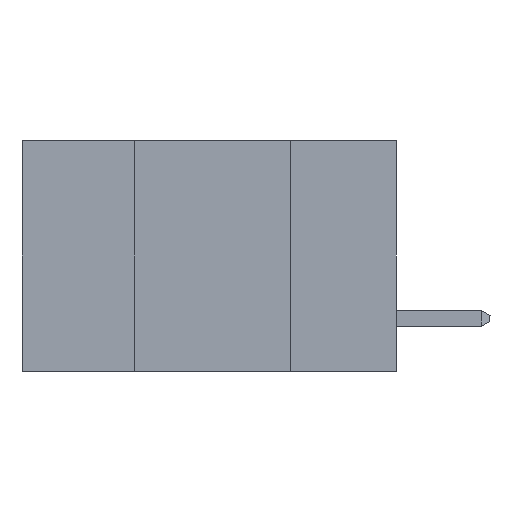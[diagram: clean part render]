
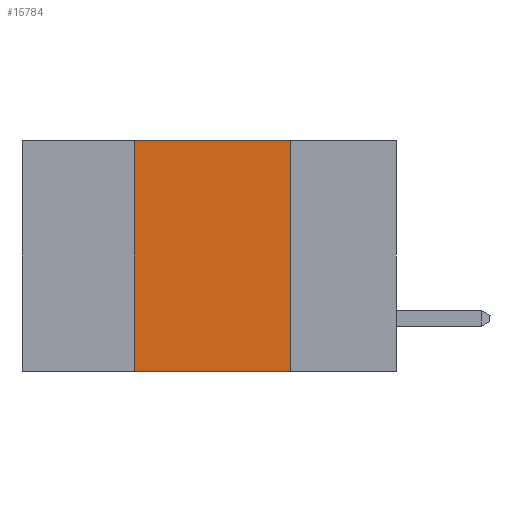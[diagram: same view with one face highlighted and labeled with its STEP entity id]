
A CAD part, left-side view. The second image highlights one B-rep face of the part: STEP entity #15784.
In plain terms, the highlighted planar face has unit normal (-1, 0, 0).
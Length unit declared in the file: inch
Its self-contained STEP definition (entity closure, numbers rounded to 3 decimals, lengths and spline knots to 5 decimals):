
#349 = DIRECTION ( 'NONE',  ( 0., 0., -1. ) ) ;
#464 = CARTESIAN_POINT ( 'NONE',  ( 0., 0.17, 0. ) ) ;
#780 = VERTEX_POINT ( 'NONE', #19838 ) ;
#867 = EDGE_CURVE ( 'NONE', #8004, #780, #4786, .T. ) ;
#2252 = VERTEX_POINT ( 'NONE', #4453 ) ;
#2405 = ORIENTED_EDGE ( 'NONE', *, *, #23906, .F. ) ;
#3900 = VECTOR ( 'NONE', #13728, 39.37008 ) ;
#4453 = CARTESIAN_POINT ( 'NONE',  ( 0., 0.42, 0. ) ) ;
#4786 = LINE ( 'NONE', #6362, #9946 ) ;
#6202 = VECTOR ( 'NONE', #10086, 39.37008 ) ;
#6362 = CARTESIAN_POINT ( 'NONE',  ( 0., 0.6, -0.37 ) ) ;
#6601 = CARTESIAN_POINT ( 'NONE',  ( 0., 0.42, -0.37 ) ) ;
#8004 = VERTEX_POINT ( 'NONE', #6601 ) ;
#8180 = PLANE ( 'NONE',  #9452 ) ;
#8631 = DIRECTION ( 'NONE',  ( 0., -1., 0. ) ) ;
#9372 = ORIENTED_EDGE ( 'NONE', *, *, #14636, .F. ) ;
#9452 = AXIS2_PLACEMENT_3D ( 'NONE', #23384, #12071, #349 ) ;
#9469 = EDGE_CURVE ( 'NONE', #20198, #780, #18580, .T. ) ;
#9946 = VECTOR ( 'NONE', #8631, 39.37008 ) ;
#10086 = DIRECTION ( 'NONE',  ( 0., -1., 0. ) ) ;
#11577 = FACE_OUTER_BOUND ( 'NONE', #12128, .T. ) ;
#12026 = DIRECTION ( 'NONE',  ( 0., 0., -1. ) ) ;
#12071 = DIRECTION ( 'NONE',  ( 1., 0., 0. ) ) ;
#12128 = EDGE_LOOP ( 'NONE', ( #14836, #2405, #9372, #17763 ) ) ;
#12157 = CARTESIAN_POINT ( 'NONE',  ( 0., 0.17, -0.37 ) ) ;
#13728 = DIRECTION ( 'NONE',  ( 0., 0., 1. ) ) ;
#14636 = EDGE_CURVE ( 'NONE', #8004, #2252, #24181, .T. ) ;
#14836 = ORIENTED_EDGE ( 'NONE', *, *, #9469, .F. ) ;
#15784 = ADVANCED_FACE ( 'NONE', ( #11577 ), #8180, .F. ) ;
#15810 = CARTESIAN_POINT ( 'NONE',  ( 0., 0.6, 0. ) ) ;
#16435 = LINE ( 'NONE', #15810, #6202 ) ;
#17763 = ORIENTED_EDGE ( 'NONE', *, *, #867, .T. ) ;
#18580 = LINE ( 'NONE', #12157, #23534 ) ;
#19453 = CARTESIAN_POINT ( 'NONE',  ( 0., 0.42, -0.37 ) ) ;
#19838 = CARTESIAN_POINT ( 'NONE',  ( 0., 0.17, -0.37 ) ) ;
#20198 = VERTEX_POINT ( 'NONE', #464 ) ;
#23384 = CARTESIAN_POINT ( 'NONE',  ( 0., 0.6, 0. ) ) ;
#23534 = VECTOR ( 'NONE', #12026, 39.37008 ) ;
#23906 = EDGE_CURVE ( 'NONE', #2252, #20198, #16435, .T. ) ;
#24181 = LINE ( 'NONE', #19453, #3900 ) ;
